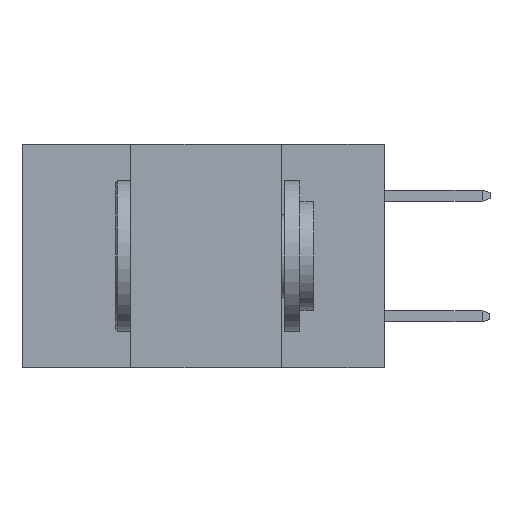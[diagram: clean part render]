
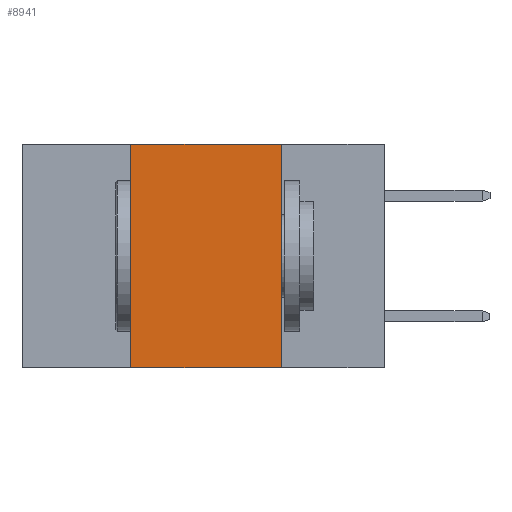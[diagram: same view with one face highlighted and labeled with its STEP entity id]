
A CAD part, left-side view. The second image highlights one B-rep face of the part: STEP entity #8941.
In plain terms, the highlighted planar face has unit normal (-1, 0, 0).
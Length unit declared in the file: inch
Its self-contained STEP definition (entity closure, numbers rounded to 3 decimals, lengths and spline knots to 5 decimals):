
#107 = LINE ( 'NONE', #6979, #2594 ) ;
#234 = CARTESIAN_POINT ( 'NONE',  ( 0., 0.42, 0. ) ) ;
#674 = DIRECTION ( 'NONE',  ( 0., 0., 1. ) ) ;
#679 = LINE ( 'NONE', #3878, #3511 ) ;
#741 = PLANE ( 'NONE',  #8640 ) ;
#1201 = DIRECTION ( 'NONE',  ( 0., -1., 0. ) ) ;
#1330 = EDGE_LOOP ( 'NONE', ( #1515, #1475, #1804, #2413 ) ) ;
#1475 = ORIENTED_EDGE ( 'NONE', *, *, #4582, .F. ) ;
#1515 = ORIENTED_EDGE ( 'NONE', *, *, #6507, .F. ) ;
#1804 = ORIENTED_EDGE ( 'NONE', *, *, #9555, .F. ) ;
#2413 = ORIENTED_EDGE ( 'NONE', *, *, #5692, .T. ) ;
#2594 = VECTOR ( 'NONE', #10588, 39.37008 ) ;
#3315 = CARTESIAN_POINT ( 'NONE',  ( 0., 0.17, 0. ) ) ;
#3511 = VECTOR ( 'NONE', #674, 39.37008 ) ;
#3878 = CARTESIAN_POINT ( 'NONE',  ( 0., 0.42, 0. ) ) ;
#4449 = LINE ( 'NONE', #7844, #9435 ) ;
#4582 = EDGE_CURVE ( 'NONE', #4613, #5205, #8957, .T. ) ;
#4613 = VERTEX_POINT ( 'NONE', #234 ) ;
#4753 = DIRECTION ( 'NONE',  ( 0., -1., 0. ) ) ;
#4951 = CARTESIAN_POINT ( 'NONE',  ( 0., 0.6, 0. ) ) ;
#5205 = VERTEX_POINT ( 'NONE', #3315 ) ;
#5692 = EDGE_CURVE ( 'NONE', #10541, #9864, #4449, .T. ) ;
#5904 = DIRECTION ( 'NONE',  ( 1., 0., 0. ) ) ;
#6319 = VECTOR ( 'NONE', #1201, 39.37008 ) ;
#6507 = EDGE_CURVE ( 'NONE', #5205, #9864, #107, .T. ) ;
#6979 = CARTESIAN_POINT ( 'NONE',  ( 0., 0.17, 0. ) ) ;
#7844 = CARTESIAN_POINT ( 'NONE',  ( 0., 0.6, -0.37 ) ) ;
#8028 = FACE_OUTER_BOUND ( 'NONE', #1330, .T. ) ;
#8640 = AXIS2_PLACEMENT_3D ( 'NONE', #4951, #5904, #12559 ) ;
#8941 = ADVANCED_FACE ( 'NONE', ( #8028 ), #741, .F. ) ;
#8957 = LINE ( 'NONE', #9950, #6319 ) ;
#9267 = CARTESIAN_POINT ( 'NONE',  ( 0., 0.17, -0.37 ) ) ;
#9435 = VECTOR ( 'NONE', #4753, 39.37008 ) ;
#9555 = EDGE_CURVE ( 'NONE', #10541, #4613, #679, .T. ) ;
#9864 = VERTEX_POINT ( 'NONE', #9267 ) ;
#9950 = CARTESIAN_POINT ( 'NONE',  ( 0., 0.6, 0. ) ) ;
#10541 = VERTEX_POINT ( 'NONE', #12721 ) ;
#10588 = DIRECTION ( 'NONE',  ( 0., 0., -1. ) ) ;
#12559 = DIRECTION ( 'NONE',  ( 0., 0., -1. ) ) ;
#12721 = CARTESIAN_POINT ( 'NONE',  ( 0., 0.42, -0.37 ) ) ;
